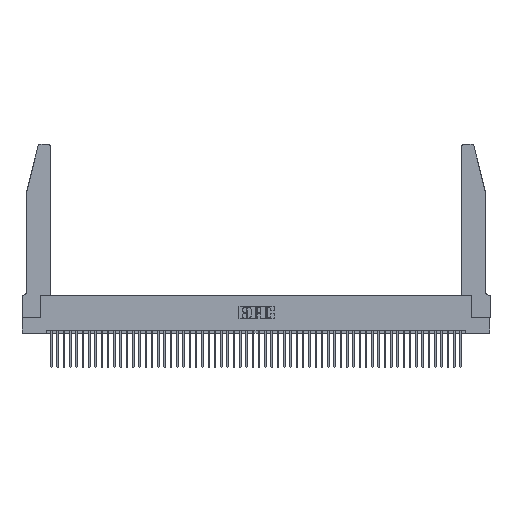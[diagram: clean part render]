
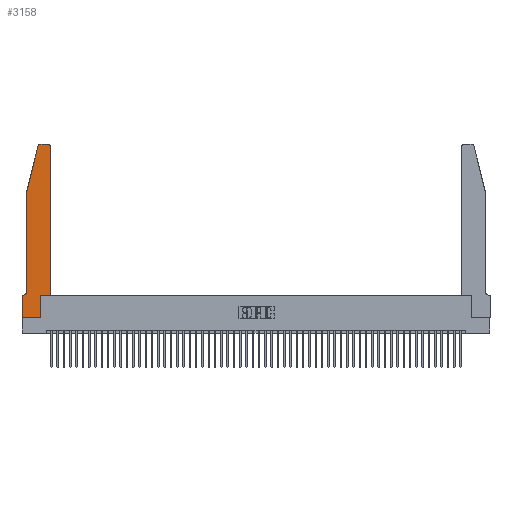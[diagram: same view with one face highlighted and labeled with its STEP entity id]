
A CAD part, top view. The second image highlights one B-rep face of the part: STEP entity #3158.
In plain terms, the highlighted planar face has unit normal (0, 0, 1).
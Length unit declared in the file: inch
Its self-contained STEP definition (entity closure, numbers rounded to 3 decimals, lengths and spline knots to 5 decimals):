
#14 = DIRECTION ( 'NONE',  ( -1., 0., 0. ) ) ;
#170 = AXIS2_PLACEMENT_3D ( 'NONE', #40559, #31956, #36611 ) ;
#535 = CARTESIAN_POINT ( 'NONE',  ( 0.2865, 0., 0.37 ) ) ;
#598 = VECTOR ( 'NONE', #47564, 39.37008 ) ;
#718 = CARTESIAN_POINT ( 'NONE',  ( 0.4205, 2.72, 0.37 ) ) ;
#2038 = CARTESIAN_POINT ( 'NONE',  ( 0.25487, 2.72718, 0.37 ) ) ;
#3158 = ADVANCED_FACE ( 'NONE', ( #35254 ), #40026, .T. ) ;
#3699 = VERTEX_POINT ( 'NONE', #29920 ) ;
#4347 = VECTOR ( 'NONE', #34404, 39.37008 ) ;
#4476 = LINE ( 'NONE', #39435, #598 ) ;
#4492 = DIRECTION ( 'NONE',  ( 0., 0., 1. ) ) ;
#4498 = LINE ( 'NONE', #15991, #24397 ) ;
#4684 = AXIS2_PLACEMENT_3D ( 'NONE', #718, #4492, #25902 ) ;
#5151 = ORIENTED_EDGE ( 'NONE', *, *, #13261, .T. ) ;
#6103 = CIRCLE ( 'NONE', #4684, 0.03 ) ;
#6200 = LINE ( 'NONE', #35451, #7466 ) ;
#6740 = EDGE_CURVE ( 'NONE', #42259, #10830, #30998, .T. ) ;
#6776 = CARTESIAN_POINT ( 'NONE',  ( 0.284, 2.75, 0.37 ) ) ;
#7096 = AXIS2_PLACEMENT_3D ( 'NONE', #15347, #40983, #14 ) ;
#7466 = VECTOR ( 'NONE', #51370, 39.37008 ) ;
#7603 = EDGE_CURVE ( 'NONE', #36492, #18658, #4498, .T. ) ;
#8070 = VECTOR ( 'NONE', #33609, 39.37008 ) ;
#9254 = ORIENTED_EDGE ( 'NONE', *, *, #38544, .T. ) ;
#10830 = VERTEX_POINT ( 'NONE', #47536 ) ;
#11038 = ORIENTED_EDGE ( 'NONE', *, *, #20228, .T. ) ;
#11666 = LINE ( 'NONE', #45020, #43164 ) ;
#12383 = VECTOR ( 'NONE', #33200, 39.37008 ) ;
#13095 = ORIENTED_EDGE ( 'NONE', *, *, #39008, .T. ) ;
#13261 = EDGE_CURVE ( 'NONE', #17377, #53038, #29887, .T. ) ;
#14001 = CARTESIAN_POINT ( 'NONE',  ( 0.0055, 0.35, 0.37 ) ) ;
#15328 = CIRCLE ( 'NONE', #23729, 0.03 ) ;
#15347 = CARTESIAN_POINT ( 'NONE',  ( 0.0055, 0.42, 0.37 ) ) ;
#15991 = CARTESIAN_POINT ( 'NONE',  ( 0.4505, 0.35, 0.37 ) ) ;
#17377 = VERTEX_POINT ( 'NONE', #40399 ) ;
#17864 = LINE ( 'NONE', #42468, #4347 ) ;
#18143 = EDGE_CURVE ( 'NONE', #18658, #24533, #51985, .T. ) ;
#18585 = EDGE_CURVE ( 'NONE', #10830, #31414, #31106, .T. ) ;
#18658 = VERTEX_POINT ( 'NONE', #53318 ) ;
#20228 = EDGE_CURVE ( 'NONE', #53038, #29694, #11666, .T. ) ;
#20530 = ORIENTED_EDGE ( 'NONE', *, *, #30576, .T. ) ;
#20543 = DIRECTION ( 'NONE',  ( 1., 0., 0. ) ) ;
#20962 = ORIENTED_EDGE ( 'NONE', *, *, #52328, .T. ) ;
#22848 = CARTESIAN_POINT ( 'NONE',  ( 0., 0., 0.37 ) ) ;
#23729 = AXIS2_PLACEMENT_3D ( 'NONE', #26562, #43081, #34993 ) ;
#24397 = VECTOR ( 'NONE', #27861, 39.37008 ) ;
#24406 = VERTEX_POINT ( 'NONE', #6776 ) ;
#24533 = VERTEX_POINT ( 'NONE', #44333 ) ;
#24535 = CARTESIAN_POINT ( 'NONE',  ( 0.4505, 0.35, 0.37 ) ) ;
#25082 = CARTESIAN_POINT ( 'NONE',  ( 0.0755, 2., 0.37 ) ) ;
#25586 = CARTESIAN_POINT ( 'NONE',  ( 0.2865, 0.35, 0.37 ) ) ;
#25902 = DIRECTION ( 'NONE',  ( 1., 0., 0. ) ) ;
#26018 = ORIENTED_EDGE ( 'NONE', *, *, #48636, .T. ) ;
#26291 = DIRECTION ( 'NONE',  ( 0., -1., 0. ) ) ;
#26562 = CARTESIAN_POINT ( 'NONE',  ( 0.284, 2.72, 0.37 ) ) ;
#26896 = VERTEX_POINT ( 'NONE', #2038 ) ;
#27112 = ORIENTED_EDGE ( 'NONE', *, *, #32660, .T. ) ;
#27141 = ORIENTED_EDGE ( 'NONE', *, *, #6740, .T. ) ;
#27801 = CARTESIAN_POINT ( 'NONE',  ( 0., 0., 0.37 ) ) ;
#27861 = DIRECTION ( 'NONE',  ( 1., 0., 0. ) ) ;
#28567 = VECTOR ( 'NONE', #26291, 39.37008 ) ;
#29468 = CARTESIAN_POINT ( 'NONE',  ( 0.0755, 0.35, 0.37 ) ) ;
#29694 = VERTEX_POINT ( 'NONE', #535 ) ;
#29887 = LINE ( 'NONE', #22848, #28567 ) ;
#29920 = CARTESIAN_POINT ( 'NONE',  ( 0.4205, 2.75, 0.37 ) ) ;
#30576 = EDGE_CURVE ( 'NONE', #24406, #26896, #15328, .T. ) ;
#30998 = LINE ( 'NONE', #25082, #12383 ) ;
#31106 = CIRCLE ( 'NONE', #7096, 0.07 ) ;
#31414 = VERTEX_POINT ( 'NONE', #14001 ) ;
#31956 = DIRECTION ( 'NONE',  ( 0., 0., 1. ) ) ;
#32660 = EDGE_CURVE ( 'NONE', #31414, #17377, #38296, .T. ) ;
#33200 = DIRECTION ( 'NONE',  ( 0., -1., 0. ) ) ;
#33609 = DIRECTION ( 'NONE',  ( -1., 0., 0. ) ) ;
#33700 = ORIENTED_EDGE ( 'NONE', *, *, #7603, .T. ) ;
#34404 = DIRECTION ( 'NONE',  ( -0.239, -0.971, 0. ) ) ;
#34993 = DIRECTION ( 'NONE',  ( 1., 0., 0. ) ) ;
#35254 = FACE_OUTER_BOUND ( 'NONE', #38210, .T. ) ;
#35451 = CARTESIAN_POINT ( 'NONE',  ( 0.2605, 2.75, 0.37 ) ) ;
#35850 = CARTESIAN_POINT ( 'NONE',  ( 0.0755, 2., 0.37 ) ) ;
#36492 = VERTEX_POINT ( 'NONE', #25586 ) ;
#36611 = DIRECTION ( 'NONE',  ( 1., 0., 0. ) ) ;
#38210 = EDGE_LOOP ( 'NONE', ( #9254, #20530, #26018, #27141, #50937, #27112, #5151, #11038, #20962, #33700, #42405, #13095 ) ) ;
#38296 = LINE ( 'NONE', #29468, #8070 ) ;
#38544 = EDGE_CURVE ( 'NONE', #3699, #24406, #6200, .T. ) ;
#39008 = EDGE_CURVE ( 'NONE', #24533, #3699, #6103, .T. ) ;
#39435 = CARTESIAN_POINT ( 'NONE',  ( 0.2865, 0.35, 0.37 ) ) ;
#40026 = PLANE ( 'NONE',  #170 ) ;
#40399 = CARTESIAN_POINT ( 'NONE',  ( 0., 0.35, 0.37 ) ) ;
#40559 = CARTESIAN_POINT ( 'NONE',  ( 0., 0.35, 0.37 ) ) ;
#40983 = DIRECTION ( 'NONE',  ( 0., 0., -1. ) ) ;
#42259 = VERTEX_POINT ( 'NONE', #35850 ) ;
#42405 = ORIENTED_EDGE ( 'NONE', *, *, #18143, .T. ) ;
#42468 = CARTESIAN_POINT ( 'NONE',  ( 0.0755, 2., 0.37 ) ) ;
#43081 = DIRECTION ( 'NONE',  ( 0., 0., 1. ) ) ;
#43164 = VECTOR ( 'NONE', #20543, 39.37008 ) ;
#44333 = CARTESIAN_POINT ( 'NONE',  ( 0.4505, 2.72, 0.37 ) ) ;
#45020 = CARTESIAN_POINT ( 'NONE',  ( 0., 0., 0.37 ) ) ;
#47536 = CARTESIAN_POINT ( 'NONE',  ( 0.0755, 0.42, 0.37 ) ) ;
#47564 = DIRECTION ( 'NONE',  ( 0., 1., 0. ) ) ;
#48636 = EDGE_CURVE ( 'NONE', #26896, #42259, #17864, .T. ) ;
#48840 = DIRECTION ( 'NONE',  ( 0., 1., 0. ) ) ;
#50937 = ORIENTED_EDGE ( 'NONE', *, *, #18585, .T. ) ;
#51313 = VECTOR ( 'NONE', #48840, 39.37008 ) ;
#51370 = DIRECTION ( 'NONE',  ( -1., 0., 0. ) ) ;
#51985 = LINE ( 'NONE', #24535, #51313 ) ;
#52328 = EDGE_CURVE ( 'NONE', #29694, #36492, #4476, .T. ) ;
#53038 = VERTEX_POINT ( 'NONE', #27801 ) ;
#53318 = CARTESIAN_POINT ( 'NONE',  ( 0.4505, 0.35, 0.37 ) ) ;
